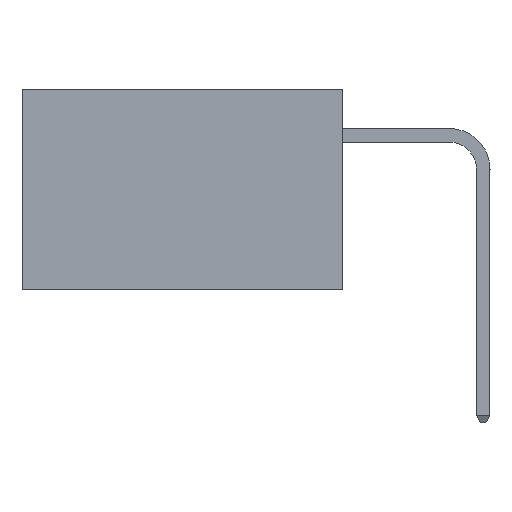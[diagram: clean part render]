
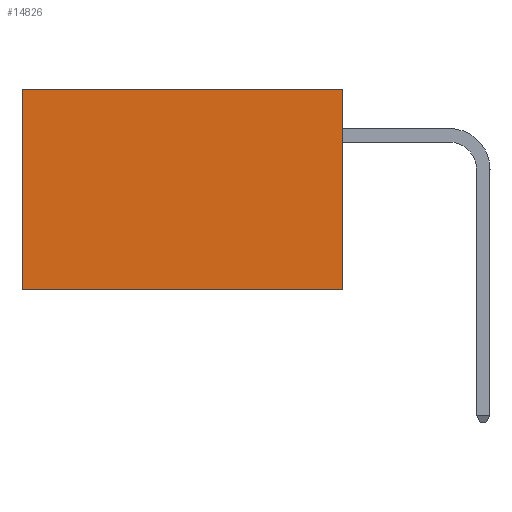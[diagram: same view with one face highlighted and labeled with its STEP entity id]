
A CAD part, left-side view. The second image highlights one B-rep face of the part: STEP entity #14826.
In plain terms, the highlighted planar face has unit normal (-1, 0, 0).
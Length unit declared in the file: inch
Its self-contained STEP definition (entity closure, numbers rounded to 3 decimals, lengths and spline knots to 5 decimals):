
#11 = LINE ( 'NONE', #5864, #10809 ) ;
#324 = DIRECTION ( 'NONE',  ( 0., 1., 0. ) ) ;
#470 = ORIENTED_EDGE ( 'NONE', *, *, #14032, .F. ) ;
#573 = EDGE_CURVE ( 'NONE', #17933, #4800, #11, .T. ) ;
#590 = ORIENTED_EDGE ( 'NONE', *, *, #5811, .T. ) ;
#741 = CARTESIAN_POINT ( 'NONE',  ( 0.277, 0.59, -0.37 ) ) ;
#836 = EDGE_LOOP ( 'NONE', ( #590, #6371, #470, #8704 ) ) ;
#912 = CARTESIAN_POINT ( 'NONE',  ( 0.277, 0.59, -0.37 ) ) ;
#1222 = VECTOR ( 'NONE', #17813, 39.37008 ) ;
#1310 = LINE ( 'NONE', #2003, #8311 ) ;
#2003 = CARTESIAN_POINT ( 'NONE',  ( 0.277, 0., -0.37 ) ) ;
#2386 = VECTOR ( 'NONE', #7427, 39.37008 ) ;
#2626 = CARTESIAN_POINT ( 'NONE',  ( 0.277, 0., -0.37 ) ) ;
#3557 = CARTESIAN_POINT ( 'NONE',  ( 0.277, 0., -0.37 ) ) ;
#3841 = AXIS2_PLACEMENT_3D ( 'NONE', #2626, #12452, #3987 ) ;
#3987 = DIRECTION ( 'NONE',  ( 0., 0., -1. ) ) ;
#4800 = VERTEX_POINT ( 'NONE', #6808 ) ;
#5811 = EDGE_CURVE ( 'NONE', #4800, #16657, #14017, .T. ) ;
#5864 = CARTESIAN_POINT ( 'NONE',  ( 0.277, 0., 0. ) ) ;
#6371 = ORIENTED_EDGE ( 'NONE', *, *, #7173, .F. ) ;
#6808 = CARTESIAN_POINT ( 'NONE',  ( 0.277, 0.59, 0. ) ) ;
#7173 = EDGE_CURVE ( 'NONE', #9669, #16657, #8237, .T. ) ;
#7427 = DIRECTION ( 'NONE',  ( 0., 0., -1. ) ) ;
#8031 = CARTESIAN_POINT ( 'NONE',  ( 0.277, 0., -0.37 ) ) ;
#8237 = LINE ( 'NONE', #8031, #1222 ) ;
#8311 = VECTOR ( 'NONE', #10418, 39.37008 ) ;
#8704 = ORIENTED_EDGE ( 'NONE', *, *, #573, .T. ) ;
#9342 = CARTESIAN_POINT ( 'NONE',  ( 0.277, 0., 0. ) ) ;
#9669 = VERTEX_POINT ( 'NONE', #3557 ) ;
#10418 = DIRECTION ( 'NONE',  ( 0., 0., -1. ) ) ;
#10809 = VECTOR ( 'NONE', #324, 39.37008 ) ;
#11065 = PLANE ( 'NONE',  #3841 ) ;
#12452 = DIRECTION ( 'NONE',  ( 1., 0., 0. ) ) ;
#13355 = FACE_OUTER_BOUND ( 'NONE', #836, .T. ) ;
#14017 = LINE ( 'NONE', #741, #2386 ) ;
#14032 = EDGE_CURVE ( 'NONE', #17933, #9669, #1310, .T. ) ;
#14826 = ADVANCED_FACE ( 'NONE', ( #13355 ), #11065, .F. ) ;
#16657 = VERTEX_POINT ( 'NONE', #912 ) ;
#17813 = DIRECTION ( 'NONE',  ( 0., 1., 0. ) ) ;
#17933 = VERTEX_POINT ( 'NONE', #9342 ) ;
